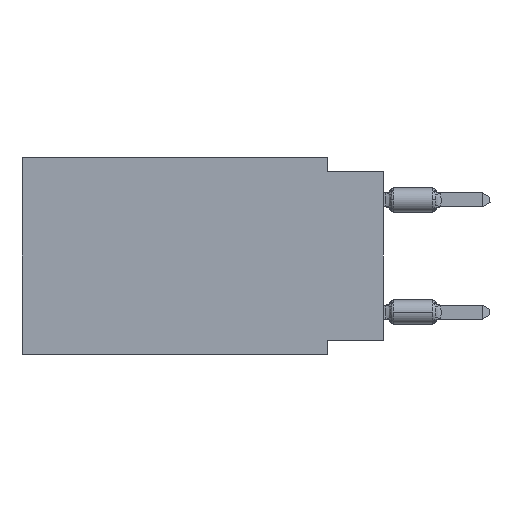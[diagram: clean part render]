
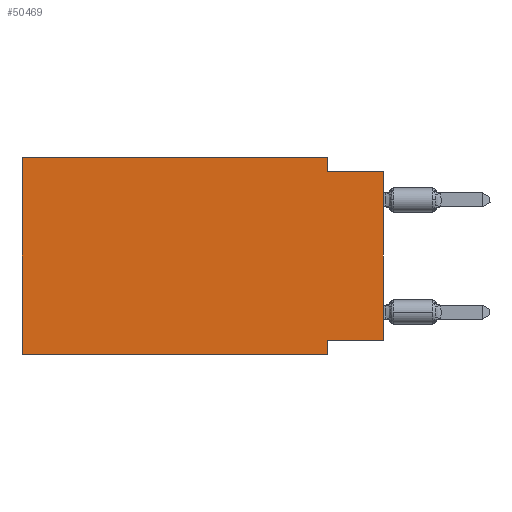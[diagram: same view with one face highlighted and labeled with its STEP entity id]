
A CAD part, left-side view. The second image highlights one B-rep face of the part: STEP entity #50469.
In plain terms, the highlighted planar face has unit normal (-1, 0, 0).
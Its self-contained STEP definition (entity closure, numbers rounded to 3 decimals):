
#456 = CARTESIAN_POINT ( 'NONE',  ( 0., 0., 0. ) ) ;
#1753 = CARTESIAN_POINT ( 'NONE',  ( 0., 0., -0.635 ) ) ;
#2616 = EDGE_LOOP ( 'NONE', ( #22485, #37800, #14529, #19508, #22870, #19188, #43881, #19275 ) ) ;
#4905 = VERTEX_POINT ( 'NONE', #42746 ) ;
#5353 = DIRECTION ( 'NONE',  ( 0., 0., -1. ) ) ;
#8776 = VERTEX_POINT ( 'NONE', #49077 ) ;
#10872 = CARTESIAN_POINT ( 'NONE',  ( 0., 16.383, 0. ) ) ;
#11703 = CARTESIAN_POINT ( 'NONE',  ( 0., 16.383, 0. ) ) ;
#13574 = VECTOR ( 'NONE', #5353, 1000. ) ;
#14014 = LINE ( 'NONE', #42514, #45342 ) ;
#14373 = VERTEX_POINT ( 'NONE', #51930 ) ;
#14469 = DIRECTION ( 'NONE',  ( 0., -1., 0. ) ) ;
#14529 = ORIENTED_EDGE ( 'NONE', *, *, #48131, .F. ) ;
#16131 = CARTESIAN_POINT ( 'NONE',  ( 0., 2.54, -8.255 ) ) ;
#18344 = LINE ( 'NONE', #1753, #47358 ) ;
#19188 = ORIENTED_EDGE ( 'NONE', *, *, #43225, .T. ) ;
#19264 = VECTOR ( 'NONE', #49597, 1000. ) ;
#19275 = ORIENTED_EDGE ( 'NONE', *, *, #33948, .F. ) ;
#19508 = ORIENTED_EDGE ( 'NONE', *, *, #31008, .F. ) ;
#19706 = CARTESIAN_POINT ( 'NONE',  ( 0., 16.383, 0. ) ) ;
#19985 = EDGE_CURVE ( 'NONE', #37497, #24602, #49864, .T. ) ;
#20529 = PLANE ( 'NONE',  #41002 ) ;
#22485 = ORIENTED_EDGE ( 'NONE', *, *, #28729, .T. ) ;
#22565 = LINE ( 'NONE', #456, #43663 ) ;
#22870 = ORIENTED_EDGE ( 'NONE', *, *, #19985, .F. ) ;
#23927 = LINE ( 'NONE', #45508, #36856 ) ;
#24237 = VECTOR ( 'NONE', #44768, 1000. ) ;
#24602 = VERTEX_POINT ( 'NONE', #10872 ) ;
#26390 = LINE ( 'NONE', #43259, #13574 ) ;
#27074 = LINE ( 'NONE', #43653, #24237 ) ;
#28729 = EDGE_CURVE ( 'NONE', #8776, #14373, #22565, .T. ) ;
#28860 = DIRECTION ( 'NONE',  ( 1., 0., 0. ) ) ;
#30602 = DIRECTION ( 'NONE',  ( 0., 0., 1. ) ) ;
#31008 = EDGE_CURVE ( 'NONE', #24602, #38198, #27074, .T. ) ;
#32767 = DIRECTION ( 'NONE',  ( 0., 1., 0. ) ) ;
#33038 = EDGE_CURVE ( 'NONE', #4905, #14373, #18344, .T. ) ;
#33687 = LINE ( 'NONE', #42010, #49777 ) ;
#33948 = EDGE_CURVE ( 'NONE', #8776, #45580, #23927, .T. ) ;
#36856 = VECTOR ( 'NONE', #32767, 1000. ) ;
#37497 = VERTEX_POINT ( 'NONE', #51517 ) ;
#37577 = CARTESIAN_POINT ( 'NONE',  ( 0., 2.54, -8.89 ) ) ;
#37800 = ORIENTED_EDGE ( 'NONE', *, *, #33038, .F. ) ;
#38117 = DIRECTION ( 'NONE',  ( 0., -1., 0. ) ) ;
#38198 = VERTEX_POINT ( 'NONE', #53155 ) ;
#39453 = DIRECTION ( 'NONE',  ( 0., 0., -1. ) ) ;
#41002 = AXIS2_PLACEMENT_3D ( 'NONE', #19706, #28860, #45733 ) ;
#41957 = VERTEX_POINT ( 'NONE', #37577 ) ;
#42010 = CARTESIAN_POINT ( 'NONE',  ( 0., 16.383, -8.89 ) ) ;
#42514 = CARTESIAN_POINT ( 'NONE',  ( 0., 2.54, -8.89 ) ) ;
#42746 = CARTESIAN_POINT ( 'NONE',  ( 0., 2.54, -0.635 ) ) ;
#43225 = EDGE_CURVE ( 'NONE', #37497, #41957, #33687, .T. ) ;
#43259 = CARTESIAN_POINT ( 'NONE',  ( 0., 2.54, 0. ) ) ;
#43653 = CARTESIAN_POINT ( 'NONE',  ( 0., 16.383, 0. ) ) ;
#43663 = VECTOR ( 'NONE', #30602, 1000. ) ;
#43881 = ORIENTED_EDGE ( 'NONE', *, *, #49013, .F. ) ;
#44768 = DIRECTION ( 'NONE',  ( 0., -1., 0. ) ) ;
#44905 = FACE_OUTER_BOUND ( 'NONE', #2616, .T. ) ;
#45342 = VECTOR ( 'NONE', #39453, 1000. ) ;
#45508 = CARTESIAN_POINT ( 'NONE',  ( 0., 0., -8.255 ) ) ;
#45580 = VERTEX_POINT ( 'NONE', #16131 ) ;
#45733 = DIRECTION ( 'NONE',  ( 0., 0., -1. ) ) ;
#47358 = VECTOR ( 'NONE', #14469, 1000. ) ;
#48131 = EDGE_CURVE ( 'NONE', #38198, #4905, #26390, .T. ) ;
#49013 = EDGE_CURVE ( 'NONE', #45580, #41957, #14014, .T. ) ;
#49077 = CARTESIAN_POINT ( 'NONE',  ( 0., 0., -8.255 ) ) ;
#49597 = DIRECTION ( 'NONE',  ( 0., 0., 1. ) ) ;
#49777 = VECTOR ( 'NONE', #38117, 1000. ) ;
#49864 = LINE ( 'NONE', #11703, #19264 ) ;
#50469 = ADVANCED_FACE ( 'NONE', ( #44905 ), #20529, .F. ) ;
#51517 = CARTESIAN_POINT ( 'NONE',  ( 0., 16.383, -8.89 ) ) ;
#51930 = CARTESIAN_POINT ( 'NONE',  ( 0., 0., -0.635 ) ) ;
#53155 = CARTESIAN_POINT ( 'NONE',  ( 0., 2.54, 0. ) ) ;
